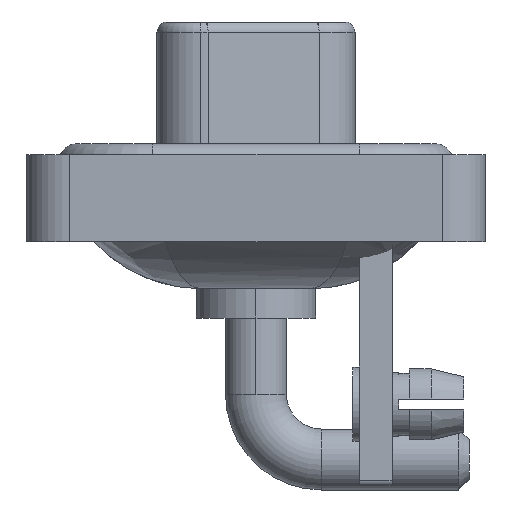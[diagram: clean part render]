
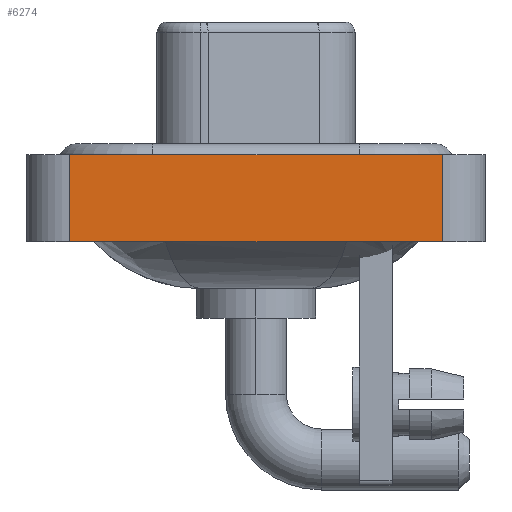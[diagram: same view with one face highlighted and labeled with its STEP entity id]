
A CAD part, left-side view. The second image highlights one B-rep face of the part: STEP entity #6274.
In plain terms, the highlighted planar face has unit normal (-1, 0, 0).
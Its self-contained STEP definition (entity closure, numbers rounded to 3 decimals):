
#28 = VECTOR ( 'NONE', #18306, 1000. ) ;
#755 = AXIS2_PLACEMENT_3D ( 'NONE', #3333, #19169, #18959 ) ;
#1037 = ORIENTED_EDGE ( 'NONE', *, *, #17413, .F. ) ;
#1191 = ORIENTED_EDGE ( 'NONE', *, *, #15958, .T. ) ;
#1380 = LINE ( 'NONE', #13993, #14480 ) ;
#2594 = CARTESIAN_POINT ( 'NONE',  ( -7.35, 8.55, -3.6 ) ) ;
#2603 = VECTOR ( 'NONE', #13750, 1000. ) ;
#2961 = VERTEX_POINT ( 'NONE', #14846 ) ;
#3236 = PLANE ( 'NONE',  #755 ) ;
#3333 = CARTESIAN_POINT ( 'NONE',  ( -7.35, -8.55, -3.6 ) ) ;
#4772 = DIRECTION ( 'NONE',  ( 0., -1., 0. ) ) ;
#5594 = EDGE_LOOP ( 'NONE', ( #1191, #10283, #1037, #16395 ) ) ;
#5993 = LINE ( 'NONE', #17182, #2603 ) ;
#6274 = ADVANCED_FACE ( 'NONE', ( #12862 ), #3236, .T. ) ;
#7153 = CARTESIAN_POINT ( 'NONE',  ( -7.35, 8.55, 0.4 ) ) ;
#7196 = EDGE_CURVE ( 'NONE', #10780, #2961, #7886, .T. ) ;
#7886 = LINE ( 'NONE', #19241, #12804 ) ;
#10283 = ORIENTED_EDGE ( 'NONE', *, *, #17207, .F. ) ;
#10780 = VERTEX_POINT ( 'NONE', #2594 ) ;
#11172 = CARTESIAN_POINT ( 'NONE',  ( -7.35, -8.55, 0.4 ) ) ;
#12568 = DIRECTION ( 'NONE',  ( 0., -1., 0. ) ) ;
#12804 = VECTOR ( 'NONE', #4772, 1000. ) ;
#12816 = VERTEX_POINT ( 'NONE', #7153 ) ;
#12862 = FACE_OUTER_BOUND ( 'NONE', #5594, .T. ) ;
#13750 = DIRECTION ( 'NONE',  ( 0., 0., 1. ) ) ;
#13993 = CARTESIAN_POINT ( 'NONE',  ( -7.35, -8.55, 0.4 ) ) ;
#14480 = VECTOR ( 'NONE', #12568, 1000. ) ;
#14846 = CARTESIAN_POINT ( 'NONE',  ( -7.35, -8.55, -3.6 ) ) ;
#15958 = EDGE_CURVE ( 'NONE', #2961, #16171, #20259, .T. ) ;
#16171 = VERTEX_POINT ( 'NONE', #11172 ) ;
#16395 = ORIENTED_EDGE ( 'NONE', *, *, #7196, .T. ) ;
#17073 = CARTESIAN_POINT ( 'NONE',  ( -7.35, -8.55, -3.6 ) ) ;
#17182 = CARTESIAN_POINT ( 'NONE',  ( -7.35, 8.55, -3.6 ) ) ;
#17207 = EDGE_CURVE ( 'NONE', #12816, #16171, #1380, .T. ) ;
#17413 = EDGE_CURVE ( 'NONE', #10780, #12816, #5993, .T. ) ;
#18306 = DIRECTION ( 'NONE',  ( 0., 0., 1. ) ) ;
#18959 = DIRECTION ( 'NONE',  ( 0., 0., 1. ) ) ;
#19169 = DIRECTION ( 'NONE',  ( -1., 0., 0. ) ) ;
#19241 = CARTESIAN_POINT ( 'NONE',  ( -7.35, -8.55, -3.6 ) ) ;
#20259 = LINE ( 'NONE', #17073, #28 ) ;
